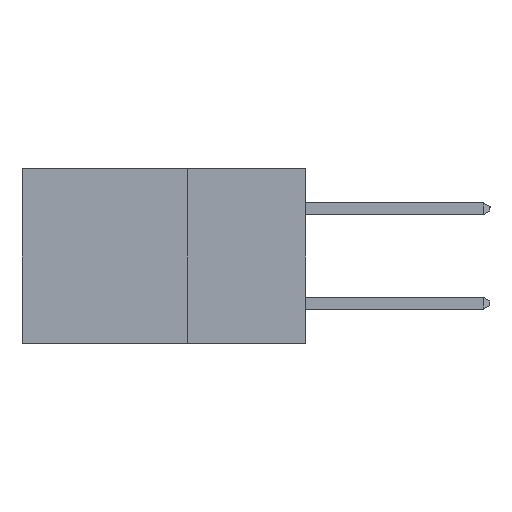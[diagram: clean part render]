
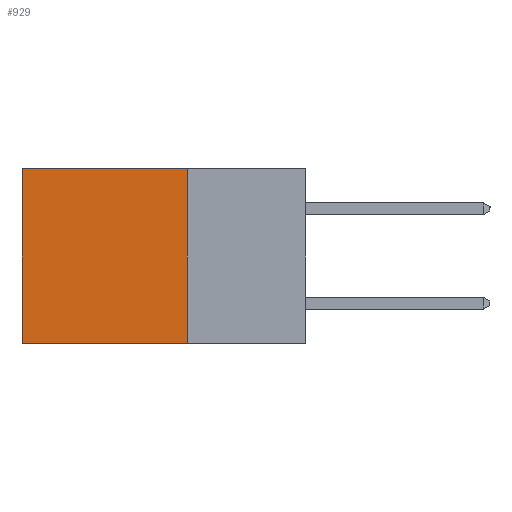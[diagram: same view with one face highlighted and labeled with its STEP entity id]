
A CAD part, left-side view. The second image highlights one B-rep face of the part: STEP entity #929.
In plain terms, the highlighted planar face has unit normal (-1, 0, 0).
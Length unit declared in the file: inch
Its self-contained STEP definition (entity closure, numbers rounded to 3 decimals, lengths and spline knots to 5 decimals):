
#929 = ADVANCED_FACE ( 'NONE', ( #8240 ), #9980, .F. ) ;
#975 = EDGE_CURVE ( 'NONE', #4642, #3977, #7625, .T. ) ;
#1018 = VERTEX_POINT ( 'NONE', #6858 ) ;
#1289 = CARTESIAN_POINT ( 'NONE',  ( 0.2615, 0.6, 0. ) ) ;
#1328 = EDGE_LOOP ( 'NONE', ( #4826, #5978, #7038, #7696 ) ) ;
#1492 = EDGE_CURVE ( 'NONE', #9138, #1018, #9919, .T. ) ;
#1942 = DIRECTION ( 'NONE',  ( 1., 0., 0. ) ) ;
#2089 = CARTESIAN_POINT ( 'NONE',  ( 0.2615, 0.6, -0.37 ) ) ;
#3400 = LINE ( 'NONE', #8146, #7612 ) ;
#3446 = DIRECTION ( 'NONE',  ( 0., 1., 0. ) ) ;
#3977 = VERTEX_POINT ( 'NONE', #8474 ) ;
#4291 = AXIS2_PLACEMENT_3D ( 'NONE', #9823, #1942, #4449 ) ;
#4449 = DIRECTION ( 'NONE',  ( 0., 0., -1. ) ) ;
#4642 = VERTEX_POINT ( 'NONE', #8861 ) ;
#4826 = ORIENTED_EDGE ( 'NONE', *, *, #1492, .T. ) ;
#4987 = LINE ( 'NONE', #5662, #8418 ) ;
#5662 = CARTESIAN_POINT ( 'NONE',  ( 0.2615, 0.25, 0. ) ) ;
#5978 = ORIENTED_EDGE ( 'NONE', *, *, #7226, .F. ) ;
#6436 = VECTOR ( 'NONE', #6596, 39.37008 ) ;
#6596 = DIRECTION ( 'NONE',  ( 0., 0., -1. ) ) ;
#6710 = DIRECTION ( 'NONE',  ( 0., 0., -1. ) ) ;
#6757 = CARTESIAN_POINT ( 'NONE',  ( 0.2615, 0.25, -0.37 ) ) ;
#6858 = CARTESIAN_POINT ( 'NONE',  ( 0.2615, 0.6, -0.37 ) ) ;
#7038 = ORIENTED_EDGE ( 'NONE', *, *, #975, .F. ) ;
#7226 = EDGE_CURVE ( 'NONE', #3977, #1018, #3400, .T. ) ;
#7612 = VECTOR ( 'NONE', #3446, 39.37008 ) ;
#7625 = LINE ( 'NONE', #6757, #9685 ) ;
#7696 = ORIENTED_EDGE ( 'NONE', *, *, #9143, .T. ) ;
#8103 = DIRECTION ( 'NONE',  ( 0., 1., 0. ) ) ;
#8146 = CARTESIAN_POINT ( 'NONE',  ( 0.2615, 0.25, -0.37 ) ) ;
#8240 = FACE_OUTER_BOUND ( 'NONE', #1328, .T. ) ;
#8418 = VECTOR ( 'NONE', #8103, 39.37008 ) ;
#8474 = CARTESIAN_POINT ( 'NONE',  ( 0.2615, 0.25, -0.37 ) ) ;
#8861 = CARTESIAN_POINT ( 'NONE',  ( 0.2615, 0.25, 0. ) ) ;
#9138 = VERTEX_POINT ( 'NONE', #1289 ) ;
#9143 = EDGE_CURVE ( 'NONE', #4642, #9138, #4987, .T. ) ;
#9685 = VECTOR ( 'NONE', #6710, 39.37008 ) ;
#9823 = CARTESIAN_POINT ( 'NONE',  ( 0.2615, 0.25, -0.37 ) ) ;
#9919 = LINE ( 'NONE', #2089, #6436 ) ;
#9980 = PLANE ( 'NONE',  #4291 ) ;
